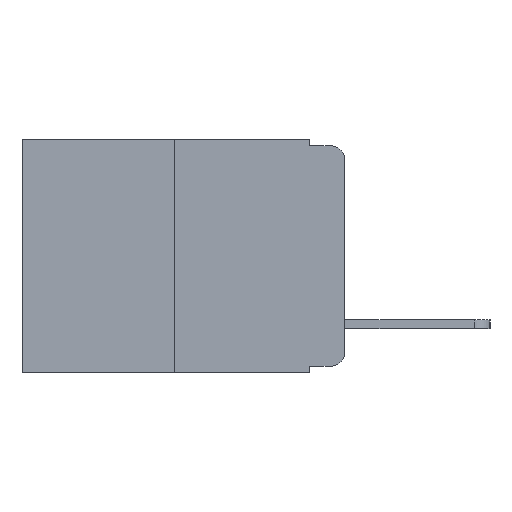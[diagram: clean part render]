
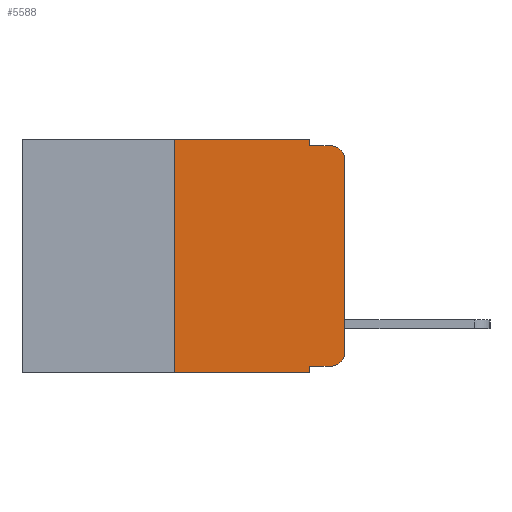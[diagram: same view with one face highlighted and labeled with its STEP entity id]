
A CAD part, left-side view. The second image highlights one B-rep face of the part: STEP entity #5588.
In plain terms, the highlighted planar face has unit normal (-1, 0, 0).
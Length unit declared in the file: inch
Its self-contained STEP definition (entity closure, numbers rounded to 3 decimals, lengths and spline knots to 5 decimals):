
#77 = DIRECTION ( 'NONE',  ( 0., 0., -1. ) ) ;
#128 = ORIENTED_EDGE ( 'NONE', *, *, #13128, .T. ) ;
#150 = VERTEX_POINT ( 'NONE', #1065 ) ;
#161 = ORIENTED_EDGE ( 'NONE', *, *, #2882, .F. ) ;
#233 = CARTESIAN_POINT ( 'NONE',  ( 0., 0.051, -0.343 ) ) ;
#395 = CARTESIAN_POINT ( 'NONE',  ( 0., 0.051, -0.333 ) ) ;
#467 = CARTESIAN_POINT ( 'NONE',  ( 0., 0.02, -0.313 ) ) ;
#680 = VERTEX_POINT ( 'NONE', #7914 ) ;
#1065 = CARTESIAN_POINT ( 'NONE',  ( 0., 0., -0.03 ) ) ;
#1292 = CARTESIAN_POINT ( 'NONE',  ( 0., 0.02, -0.03 ) ) ;
#1401 = EDGE_CURVE ( 'NONE', #150, #8309, #6709, .T. ) ;
#1562 = DIRECTION ( 'NONE',  ( 0., 0., 1. ) ) ;
#1575 = DIRECTION ( 'NONE',  ( 0., 0., -1. ) ) ;
#1632 = VECTOR ( 'NONE', #8444, 39.37008 ) ;
#1696 = VECTOR ( 'NONE', #1562, 39.37008 ) ;
#2572 = ORIENTED_EDGE ( 'NONE', *, *, #9610, .F. ) ;
#2681 = PLANE ( 'NONE',  #9554 ) ;
#2882 = EDGE_CURVE ( 'NONE', #13511, #7229, #13098, .T. ) ;
#2897 = DIRECTION ( 'NONE',  ( 0., 0., -1. ) ) ;
#3226 = EDGE_CURVE ( 'NONE', #9925, #10613, #8883, .T. ) ;
#3415 = ORIENTED_EDGE ( 'NONE', *, *, #5569, .T. ) ;
#3767 = DIRECTION ( 'NONE',  ( 0., -1., 0. ) ) ;
#3805 = DIRECTION ( 'NONE',  ( 1., 0., 0. ) ) ;
#3863 = CARTESIAN_POINT ( 'NONE',  ( 0., 0.051, 0. ) ) ;
#3995 = CARTESIAN_POINT ( 'NONE',  ( 0., 0.02, -0.01 ) ) ;
#4150 = ORIENTED_EDGE ( 'NONE', *, *, #9398, .T. ) ;
#4336 = ORIENTED_EDGE ( 'NONE', *, *, #13792, .F. ) ;
#4599 = LINE ( 'NONE', #13788, #1632 ) ;
#4607 = DIRECTION ( 'NONE',  ( -1., 0., 0. ) ) ;
#4671 = ORIENTED_EDGE ( 'NONE', *, *, #7887, .F. ) ;
#5082 = VECTOR ( 'NONE', #8537, 39.37008 ) ;
#5131 = LINE ( 'NONE', #395, #5476 ) ;
#5266 = LINE ( 'NONE', #9240, #10402 ) ;
#5425 = AXIS2_PLACEMENT_3D ( 'NONE', #1292, #4607, #77 ) ;
#5458 = CARTESIAN_POINT ( 'NONE',  ( 0., 0.051, -0.333 ) ) ;
#5476 = VECTOR ( 'NONE', #9208, 39.37008 ) ;
#5569 = EDGE_CURVE ( 'NONE', #10952, #12149, #11559, .T. ) ;
#5588 = ADVANCED_FACE ( 'NONE', ( #8328 ), #2681, .F. ) ;
#5768 = LINE ( 'NONE', #7461, #5082 ) ;
#5970 = VECTOR ( 'NONE', #13086, 39.37008 ) ;
#5983 = CARTESIAN_POINT ( 'NONE',  ( 0., 0.473, 0. ) ) ;
#6187 = CARTESIAN_POINT ( 'NONE',  ( 0., 0.25, 0. ) ) ;
#6218 = ORIENTED_EDGE ( 'NONE', *, *, #3226, .F. ) ;
#6262 = EDGE_LOOP ( 'NONE', ( #12362, #8800, #2572, #4336, #4671, #6218, #4150, #161, #128, #3415 ) ) ;
#6636 = AXIS2_PLACEMENT_3D ( 'NONE', #467, #8199, #1575 ) ;
#6709 = CIRCLE ( 'NONE', #5425, 0.02 ) ;
#7229 = VERTEX_POINT ( 'NONE', #233 ) ;
#7461 = CARTESIAN_POINT ( 'NONE',  ( 0., 0.051, -0.01 ) ) ;
#7582 = LINE ( 'NONE', #13066, #10472 ) ;
#7769 = VERTEX_POINT ( 'NONE', #13851 ) ;
#7862 = CARTESIAN_POINT ( 'NONE',  ( 0., 0.25, 0. ) ) ;
#7887 = EDGE_CURVE ( 'NONE', #10613, #680, #7582, .T. ) ;
#7914 = CARTESIAN_POINT ( 'NONE',  ( 0., 0.051, 0. ) ) ;
#8199 = DIRECTION ( 'NONE',  ( -1., 0., 0. ) ) ;
#8309 = VERTEX_POINT ( 'NONE', #3995 ) ;
#8311 = CARTESIAN_POINT ( 'NONE',  ( 0., 0., -0.313 ) ) ;
#8328 = FACE_OUTER_BOUND ( 'NONE', #6262, .T. ) ;
#8444 = DIRECTION ( 'NONE',  ( 0., 0., -1. ) ) ;
#8537 = DIRECTION ( 'NONE',  ( 0., -1., 0. ) ) ;
#8800 = ORIENTED_EDGE ( 'NONE', *, *, #1401, .T. ) ;
#8883 = LINE ( 'NONE', #6187, #5970 ) ;
#9208 = DIRECTION ( 'NONE',  ( 0., -1., 0. ) ) ;
#9240 = CARTESIAN_POINT ( 'NONE',  ( 0., 0.473, -0.343 ) ) ;
#9398 = EDGE_CURVE ( 'NONE', #9925, #7229, #5266, .T. ) ;
#9554 = AXIS2_PLACEMENT_3D ( 'NONE', #5983, #3805, #11484 ) ;
#9610 = EDGE_CURVE ( 'NONE', #7769, #8309, #5768, .T. ) ;
#9905 = VECTOR ( 'NONE', #2897, 39.37008 ) ;
#9925 = VERTEX_POINT ( 'NONE', #11236 ) ;
#10402 = VECTOR ( 'NONE', #3767, 39.37008 ) ;
#10472 = VECTOR ( 'NONE', #10929, 39.37008 ) ;
#10613 = VERTEX_POINT ( 'NONE', #7862 ) ;
#10929 = DIRECTION ( 'NONE',  ( 0., -1., 0. ) ) ;
#10952 = VERTEX_POINT ( 'NONE', #13871 ) ;
#11236 = CARTESIAN_POINT ( 'NONE',  ( 0., 0.25, -0.343 ) ) ;
#11410 = EDGE_CURVE ( 'NONE', #12149, #150, #13318, .T. ) ;
#11484 = DIRECTION ( 'NONE',  ( 0., 0., -1. ) ) ;
#11559 = CIRCLE ( 'NONE', #6636, 0.02 ) ;
#12149 = VERTEX_POINT ( 'NONE', #8311 ) ;
#12362 = ORIENTED_EDGE ( 'NONE', *, *, #11410, .T. ) ;
#13066 = CARTESIAN_POINT ( 'NONE',  ( 0., 0.473, 0. ) ) ;
#13086 = DIRECTION ( 'NONE',  ( 0., 0., 1. ) ) ;
#13098 = LINE ( 'NONE', #3863, #9905 ) ;
#13128 = EDGE_CURVE ( 'NONE', #13511, #10952, #5131, .T. ) ;
#13318 = LINE ( 'NONE', #13536, #1696 ) ;
#13511 = VERTEX_POINT ( 'NONE', #5458 ) ;
#13536 = CARTESIAN_POINT ( 'NONE',  ( 0., 0., 0. ) ) ;
#13788 = CARTESIAN_POINT ( 'NONE',  ( 0., 0.051, 0. ) ) ;
#13792 = EDGE_CURVE ( 'NONE', #680, #7769, #4599, .T. ) ;
#13851 = CARTESIAN_POINT ( 'NONE',  ( 0., 0.051, -0.01 ) ) ;
#13871 = CARTESIAN_POINT ( 'NONE',  ( 0., 0.02, -0.333 ) ) ;
